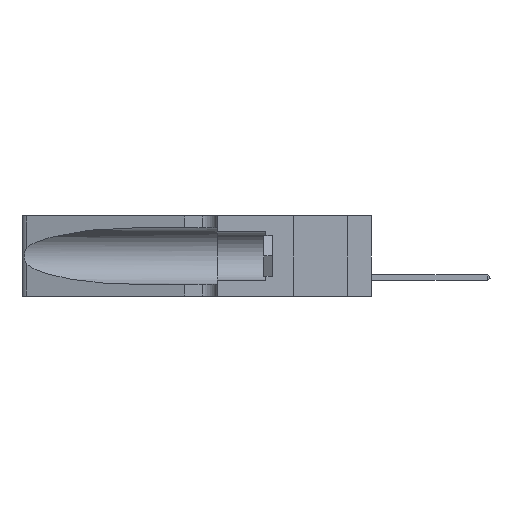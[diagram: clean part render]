
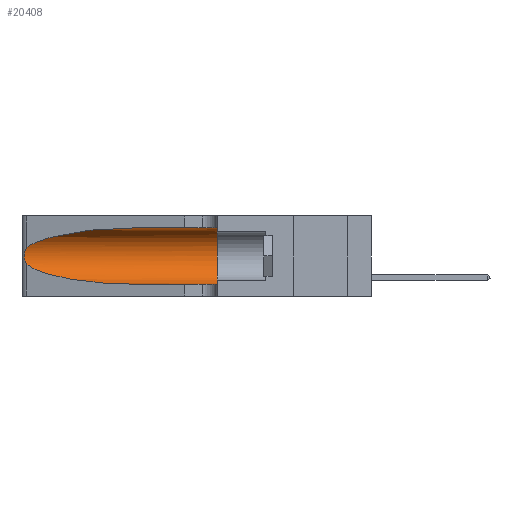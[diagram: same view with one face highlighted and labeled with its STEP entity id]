
A CAD part, left-side view. The second image highlights one B-rep face of the part: STEP entity #20408.
In plain terms, the highlighted cylindrical face has radius 3.308 mm (diameter 6.617 mm), a partial arc.
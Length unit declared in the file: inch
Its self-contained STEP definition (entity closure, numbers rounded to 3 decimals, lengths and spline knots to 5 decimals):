
#81 = VERTEX_POINT ( 'NONE', #19485 ) ;
#182 = EDGE_LOOP ( 'NONE', ( #18300, #10756, #19482, #4233, #13568, #1882 ) ) ;
#198 = VERTEX_POINT ( 'NONE', #24561 ) ;
#1805 = CARTESIAN_POINT ( 'NONE',  ( 0.25789, 1.23486, 0.15765 ) ) ;
#1882 = ORIENTED_EDGE ( 'NONE', *, *, #18345, .F. ) ;
#1943 = CARTESIAN_POINT ( 'NONE',  ( 0.26075, 1.23896, 0.19203 ) ) ;
#3137 = CARTESIAN_POINT ( 'NONE',  ( 0.1305, 0.72297, 0.31525 ) ) ;
#3324 = EDGE_CURVE ( 'NONE', #7286, #6044, #3635, .T. ) ;
#3488 = CARTESIAN_POINT ( 'NONE',  ( 0.1305, 0.35, 0.05475 ) ) ;
#3635 = LINE ( 'NONE', #35836, #27811 ) ;
#4233 = ORIENTED_EDGE ( 'NONE', *, *, #3324, .T. ) ;
#4798 = CARTESIAN_POINT ( 'NONE',  ( 0.25555, 1.22994, 0.2215 ) ) ;
#5999 = CARTESIAN_POINT ( 'NONE',  ( 0.25487, 1.22718, 0.22369 ) ) ;
#6044 = VERTEX_POINT ( 'NONE', #3488 ) ;
#6120 = VECTOR ( 'NONE', #22285, 39.37008 ) ;
#6574 = CARTESIAN_POINT ( 'NONE',  ( 0.1305, 1.61858, 0.185 ) ) ;
#6577 = CARTESIAN_POINT ( 'NONE',  ( 0.18966, 0.96281, 0.05475 ) ) ;
#7286 = VERTEX_POINT ( 'NONE', #11032 ) ;
#7685 = CARTESIAN_POINT ( 'NONE',  ( 0.25856, 1.23593, 0.16098 ) ) ;
#7799 = CARTESIAN_POINT ( 'NONE',  ( 0.25854, 1.2359, 0.20912 ) ) ;
#7836 = CYLINDRICAL_SURFACE ( 'NONE', #24953, 0.13025 ) ;
#7953 = LINE ( 'NONE', #16158, #6120 ) ;
#9571 = DIRECTION ( 'NONE',  ( 0., -1., 0. ) ) ;
#9995 = AXIS2_PLACEMENT_3D ( 'NONE', #29782, #18483, #32660 ) ;
#10288 = CARTESIAN_POINT ( 'NONE',  ( 0.25639, 1.23186, 0.15144 ) ) ;
#10536 = CARTESIAN_POINT ( 'NONE',  ( 0.26017, 1.23833, 0.17102 ) ) ;
#10756 = ORIENTED_EDGE ( 'NONE', *, *, #21571, .T. ) ;
#11032 = CARTESIAN_POINT ( 'NONE',  ( 0.1305, 0.72297, 0.05475 ) ) ;
#11264 = CARTESIAN_POINT ( 'NONE',  ( 0.18966, 0.96281, 0.31525 ) ) ;
#13002 = CARTESIAN_POINT ( 'NONE',  ( 0.25555, 1.22993, 0.14849 ) ) ;
#13568 = ORIENTED_EDGE ( 'NONE', *, *, #28296, .F. ) ;
#15913 = CARTESIAN_POINT ( 'NONE',  ( 0.25639, 1.23184, 0.21858 ) ) ;
#16158 = CARTESIAN_POINT ( 'NONE',  ( 0.1305, 1.61858, 0.31525 ) ) ;
#18300 = ORIENTED_EDGE ( 'NONE', *, *, #35252, .T. ) ;
#18345 = EDGE_CURVE ( 'NONE', #81, #30787, #7953, .T. ) ;
#18483 = DIRECTION ( 'NONE',  ( 0., 1., 0. ) ) ;
#18982 = CARTESIAN_POINT ( 'NONE',  ( 0.25787, 1.23484, 0.2124 ) ) ;
#19304 = CIRCLE ( 'NONE', #9995, 0.13025 ) ;
#19482 = ORIENTED_EDGE ( 'NONE', *, *, #33327, .T. ) ;
#19485 = CARTESIAN_POINT ( 'NONE',  ( 0.1305, 0.72297, 0.31525 ) ) ;
#20408 = ADVANCED_FACE ( 'NONE', ( #31933 ), #7836, .F. ) ;
#21571 = EDGE_CURVE ( 'NONE', #198, #24014, #30412, .T. ) ;
#22285 = DIRECTION ( 'NONE',  ( 0., -1., 0. ) ) ;
#22673 = CARTESIAN_POINT ( 'NONE',  ( 0.2373, 1.15595, 0.08982 ) ) ;
#23121 = CARTESIAN_POINT ( 'NONE',  ( 0.2373, 1.15595, 0.28018 ) ) ;
#23168 = CARTESIAN_POINT ( 'NONE',  ( 0.1305, 0.35, 0.31525 ) ) ;
#23826 = CARTESIAN_POINT ( 'NONE',  ( 0.1305, 0.72297, 0.05475 ) ) ;
#24014 = VERTEX_POINT ( 'NONE', #35742 ) ;
#24561 = CARTESIAN_POINT ( 'NONE',  ( 0.25487, 1.22718, 0.22369 ) ) ;
#24794 = CARTESIAN_POINT ( 'NONE',  ( 0.26075, 1.23896, 0.178 ) ) ;
#24924 = CARTESIAN_POINT ( 'NONE',  ( 0.26018, 1.23835, 0.19895 ) ) ;
#24953 = AXIS2_PLACEMENT_3D ( 'NONE', #6574, #9571, #29417 ) ;
#25669 = CARTESIAN_POINT ( 'NONE',  ( 0.25487, 1.22718, 0.14631 ) ) ;
#27780 = CARTESIAN_POINT ( 'NONE',  ( 0.25487, 1.22718, 0.14631 ) ) ;
#27811 = VECTOR ( 'NONE', #32939, 39.37008 ) ;
#28296 = EDGE_CURVE ( 'NONE', #30787, #6044, #19304, .T. ) ;
#29417 = DIRECTION ( 'NONE',  ( 0., 0., -1. ) ) ;
#29661 =( BOUNDED_CURVE ( )  B_SPLINE_CURVE ( 3, ( #3137, #11264, #23121, #5999 ),
 .UNSPECIFIED., .F., .F. ) 
 B_SPLINE_CURVE_WITH_KNOTS ( ( 4, 4 ),
 ( 1.5708, 2.84003 ),
 .UNSPECIFIED. ) 
 CURVE ( )  GEOMETRIC_REPRESENTATION_ITEM ( )  RATIONAL_B_SPLINE_CURVE ( ( 1., 0.87, 0.87, 1. ) ) 
 REPRESENTATION_ITEM ( '' )  );
#29782 = CARTESIAN_POINT ( 'NONE',  ( 0.1305, 0.35, 0.185 ) ) ;
#30412 = B_SPLINE_CURVE_WITH_KNOTS ( 'NONE', 3,
 ( #36044, #4798, #15913, #18982, #7799, #24924, #1943, #24794, #10536, #7685, #1805, #10288, #13002, #27780 ),
 .UNSPECIFIED., .F., .F.,
 ( 4, 2, 2, 2, 2, 2, 4 ),
 ( 0., 0.00027, 0.00053, 0.00107, 0.0016, 0.00187, 0.00214 ),
 .UNSPECIFIED. ) ;
#30787 = VERTEX_POINT ( 'NONE', #23168 ) ;
#31933 = FACE_OUTER_BOUND ( 'NONE', #182, .T. ) ;
#32660 = DIRECTION ( 'NONE',  ( 0., 0., 1. ) ) ;
#32939 = DIRECTION ( 'NONE',  ( 0., -1., 0. ) ) ;
#33327 = EDGE_CURVE ( 'NONE', #24014, #7286, #34698, .T. ) ;
#34698 =( BOUNDED_CURVE ( )  B_SPLINE_CURVE ( 3, ( #25669, #22673, #6577, #23826 ),
 .UNSPECIFIED., .F., .F. ) 
 B_SPLINE_CURVE_WITH_KNOTS ( ( 4, 4 ),
 ( 3.44316, 4.71239 ),
 .UNSPECIFIED. ) 
 CURVE ( )  GEOMETRIC_REPRESENTATION_ITEM ( )  RATIONAL_B_SPLINE_CURVE ( ( 1., 0.87, 0.87, 1. ) ) 
 REPRESENTATION_ITEM ( '' )  );
#35252 = EDGE_CURVE ( 'NONE', #81, #198, #29661, .T. ) ;
#35742 = CARTESIAN_POINT ( 'NONE',  ( 0.25487, 1.22718, 0.14631 ) ) ;
#35836 = CARTESIAN_POINT ( 'NONE',  ( 0.1305, 1.61858, 0.05475 ) ) ;
#36044 = CARTESIAN_POINT ( 'NONE',  ( 0.25487, 1.22718, 0.22369 ) ) ;
